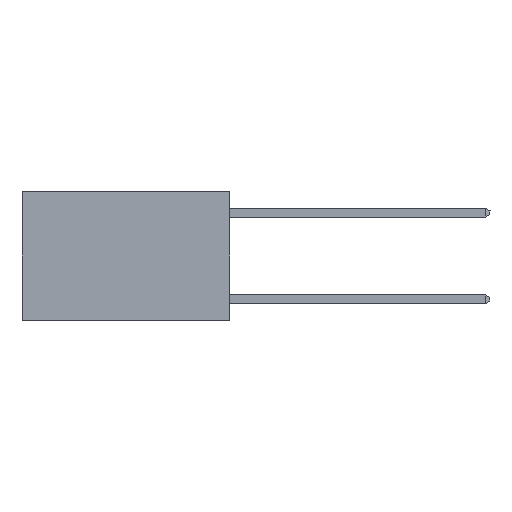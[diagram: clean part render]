
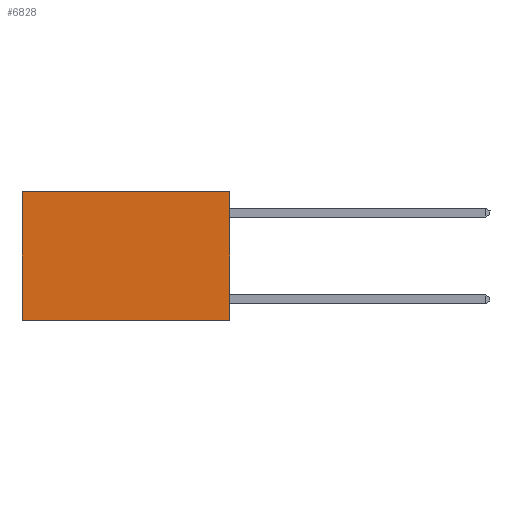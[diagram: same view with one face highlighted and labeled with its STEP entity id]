
A CAD part, left-side view. The second image highlights one B-rep face of the part: STEP entity #6828.
In plain terms, the highlighted planar face has unit normal (-1, 0, 0).
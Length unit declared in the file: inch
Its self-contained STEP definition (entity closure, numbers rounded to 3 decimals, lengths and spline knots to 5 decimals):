
#38 = CARTESIAN_POINT ( 'NONE',  ( 0.2625, 0., 0. ) ) ;
#325 = CARTESIAN_POINT ( 'NONE',  ( 0.2625, 0., 0. ) ) ;
#430 = ORIENTED_EDGE ( 'NONE', *, *, #6053, .T. ) ;
#1039 = CARTESIAN_POINT ( 'NONE',  ( 0.2625, 0.6, 0. ) ) ;
#1911 = DIRECTION ( 'NONE',  ( 0., 0., -1. ) ) ;
#2551 = LINE ( 'NONE', #3695, #4752 ) ;
#2578 = CARTESIAN_POINT ( 'NONE',  ( 0.2625, 0.6, 0. ) ) ;
#2690 = CARTESIAN_POINT ( 'NONE',  ( 0.2625, 0., -0.37 ) ) ;
#2826 = VERTEX_POINT ( 'NONE', #8760 ) ;
#2923 = DIRECTION ( 'NONE',  ( 1., 0., 0. ) ) ;
#2950 = EDGE_LOOP ( 'NONE', ( #8883, #5288, #10516, #430 ) ) ;
#3695 = CARTESIAN_POINT ( 'NONE',  ( 0.2625, 0., 0. ) ) ;
#3756 = LINE ( 'NONE', #38, #8591 ) ;
#4085 = VECTOR ( 'NONE', #1911, 39.37008 ) ;
#4313 = VERTEX_POINT ( 'NONE', #2578 ) ;
#4331 = LINE ( 'NONE', #1039, #4085 ) ;
#4701 = CARTESIAN_POINT ( 'NONE',  ( 0.2625, 0., -0.37 ) ) ;
#4752 = VECTOR ( 'NONE', #9344, 39.37008 ) ;
#5288 = ORIENTED_EDGE ( 'NONE', *, *, #6379, .F. ) ;
#5458 = EDGE_CURVE ( 'NONE', #2826, #7976, #2551, .T. ) ;
#5497 = DIRECTION ( 'NONE',  ( 0., 1., 0. ) ) ;
#5874 = AXIS2_PLACEMENT_3D ( 'NONE', #325, #2923, #8665 ) ;
#6053 = EDGE_CURVE ( 'NONE', #2826, #4313, #3756, .T. ) ;
#6379 = EDGE_CURVE ( 'NONE', #7976, #9537, #8582, .T. ) ;
#6683 = CARTESIAN_POINT ( 'NONE',  ( 0.2625, 0.6, -0.37 ) ) ;
#6828 = ADVANCED_FACE ( 'NONE', ( #7278 ), #10159, .F. ) ;
#7278 = FACE_OUTER_BOUND ( 'NONE', #2950, .T. ) ;
#7976 = VERTEX_POINT ( 'NONE', #2690 ) ;
#7995 = EDGE_CURVE ( 'NONE', #4313, #9537, #4331, .T. ) ;
#8402 = DIRECTION ( 'NONE',  ( 0., 1., 0. ) ) ;
#8582 = LINE ( 'NONE', #4701, #10120 ) ;
#8591 = VECTOR ( 'NONE', #8402, 39.37008 ) ;
#8665 = DIRECTION ( 'NONE',  ( 0., 0., -1. ) ) ;
#8760 = CARTESIAN_POINT ( 'NONE',  ( 0.2625, 0., 0. ) ) ;
#8883 = ORIENTED_EDGE ( 'NONE', *, *, #7995, .T. ) ;
#9344 = DIRECTION ( 'NONE',  ( 0., 0., -1. ) ) ;
#9537 = VERTEX_POINT ( 'NONE', #6683 ) ;
#10120 = VECTOR ( 'NONE', #5497, 39.37008 ) ;
#10159 = PLANE ( 'NONE',  #5874 ) ;
#10516 = ORIENTED_EDGE ( 'NONE', *, *, #5458, .F. ) ;
